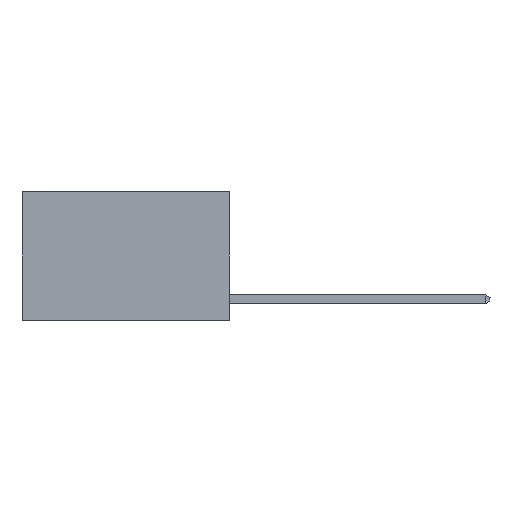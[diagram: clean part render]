
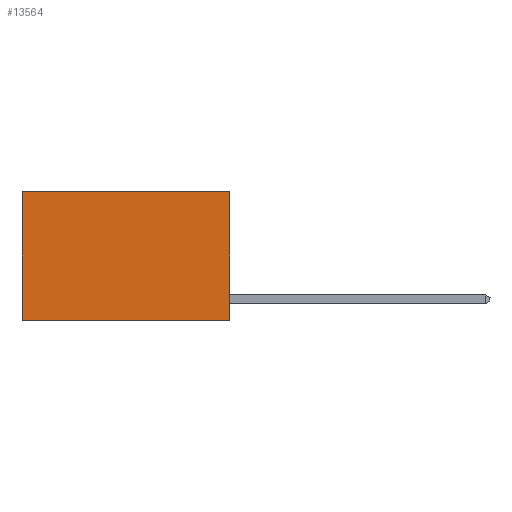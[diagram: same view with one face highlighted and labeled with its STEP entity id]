
A CAD part, left-side view. The second image highlights one B-rep face of the part: STEP entity #13564.
In plain terms, the highlighted planar face has unit normal (-1, 0, 0).
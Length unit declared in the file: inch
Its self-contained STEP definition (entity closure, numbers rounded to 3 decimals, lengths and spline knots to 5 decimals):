
#56 = VECTOR ( 'NONE', #7437, 39.37008 ) ;
#232 = PLANE ( 'NONE',  #2998 ) ;
#510 = EDGE_CURVE ( 'NONE', #2418, #7317, #9951, .T. ) ;
#835 = EDGE_LOOP ( 'NONE', ( #11648, #1850, #6401, #6530 ) ) ;
#1372 = DIRECTION ( 'NONE',  ( 0., 0., -1. ) ) ;
#1850 = ORIENTED_EDGE ( 'NONE', *, *, #5723, .F. ) ;
#2037 = EDGE_CURVE ( 'NONE', #2418, #5127, #11839, .T. ) ;
#2236 = DIRECTION ( 'NONE',  ( 0., 1., 0. ) ) ;
#2418 = VERTEX_POINT ( 'NONE', #7747 ) ;
#2998 = AXIS2_PLACEMENT_3D ( 'NONE', #12358, #8161, #1372 ) ;
#3152 = FACE_OUTER_BOUND ( 'NONE', #835, .T. ) ;
#3248 = CARTESIAN_POINT ( 'NONE',  ( 0.2625, 0.6, 0. ) ) ;
#3508 = DIRECTION ( 'NONE',  ( 0., 0., -1. ) ) ;
#3905 = VECTOR ( 'NONE', #3508, 39.37008 ) ;
#4804 = DIRECTION ( 'NONE',  ( 0., 0., -1. ) ) ;
#5127 = VERTEX_POINT ( 'NONE', #3248 ) ;
#5723 = EDGE_CURVE ( 'NONE', #7317, #13277, #12583, .T. ) ;
#6401 = ORIENTED_EDGE ( 'NONE', *, *, #510, .F. ) ;
#6530 = ORIENTED_EDGE ( 'NONE', *, *, #2037, .T. ) ;
#7317 = VERTEX_POINT ( 'NONE', #8739 ) ;
#7437 = DIRECTION ( 'NONE',  ( 0., 1., 0. ) ) ;
#7747 = CARTESIAN_POINT ( 'NONE',  ( 0.2625, 0., 0. ) ) ;
#8161 = DIRECTION ( 'NONE',  ( 1., 0., 0. ) ) ;
#8739 = CARTESIAN_POINT ( 'NONE',  ( 0.2625, 0., -0.37 ) ) ;
#9302 = CARTESIAN_POINT ( 'NONE',  ( 0.2625, 0., 0. ) ) ;
#9491 = LINE ( 'NONE', #13291, #3905 ) ;
#9628 = VECTOR ( 'NONE', #4804, 39.37008 ) ;
#9951 = LINE ( 'NONE', #9302, #9628 ) ;
#11648 = ORIENTED_EDGE ( 'NONE', *, *, #13519, .T. ) ;
#11733 = CARTESIAN_POINT ( 'NONE',  ( 0.2625, 0., 0. ) ) ;
#11839 = LINE ( 'NONE', #11733, #56 ) ;
#12262 = VECTOR ( 'NONE', #2236, 39.37008 ) ;
#12358 = CARTESIAN_POINT ( 'NONE',  ( 0.2625, 0., 0. ) ) ;
#12583 = LINE ( 'NONE', #14137, #12262 ) ;
#13277 = VERTEX_POINT ( 'NONE', #13874 ) ;
#13291 = CARTESIAN_POINT ( 'NONE',  ( 0.2625, 0.6, 0. ) ) ;
#13519 = EDGE_CURVE ( 'NONE', #5127, #13277, #9491, .T. ) ;
#13564 = ADVANCED_FACE ( 'NONE', ( #3152 ), #232, .F. ) ;
#13874 = CARTESIAN_POINT ( 'NONE',  ( 0.2625, 0.6, -0.37 ) ) ;
#14137 = CARTESIAN_POINT ( 'NONE',  ( 0.2625, 0., -0.37 ) ) ;
